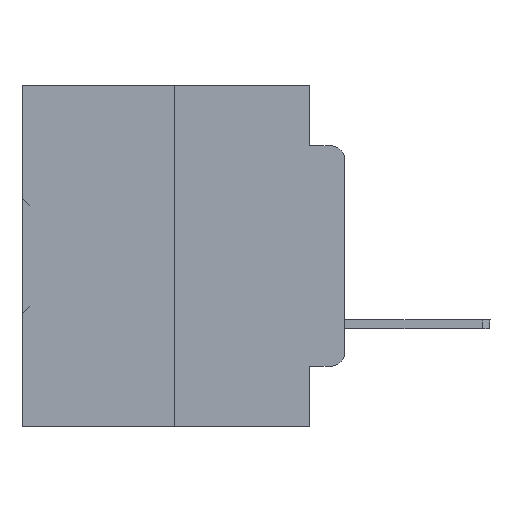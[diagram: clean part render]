
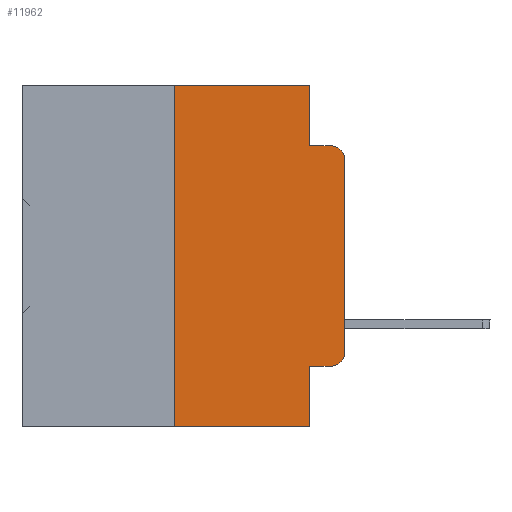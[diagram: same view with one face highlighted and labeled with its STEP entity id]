
A CAD part, left-side view. The second image highlights one B-rep face of the part: STEP entity #11962.
In plain terms, the highlighted planar face has unit normal (-1, 0, 0).
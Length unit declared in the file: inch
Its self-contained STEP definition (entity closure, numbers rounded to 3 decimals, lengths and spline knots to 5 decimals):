
#7 = PLANE ( 'NONE',  #31530 ) ;
#831 = VERTEX_POINT ( 'NONE', #22939 ) ;
#1155 = CARTESIAN_POINT ( 'NONE',  ( 0., 0.051, 0. ) ) ;
#1368 = EDGE_CURVE ( 'NONE', #8319, #36062, #19112, .T. ) ;
#2405 = DIRECTION ( 'NONE',  ( 0., 0., 1. ) ) ;
#2536 = DIRECTION ( 'NONE',  ( -1., 0., 0. ) ) ;
#2667 = CARTESIAN_POINT ( 'NONE',  ( 0., 0.051, -0.4115 ) ) ;
#2795 = LINE ( 'NONE', #1155, #24712 ) ;
#2955 = LINE ( 'NONE', #13779, #24870 ) ;
#3043 = ORIENTED_EDGE ( 'NONE', *, *, #25384, .F. ) ;
#3349 = VECTOR ( 'NONE', #2405, 39.37008 ) ;
#3354 = CARTESIAN_POINT ( 'NONE',  ( 0., 0.02, -0.0885 ) ) ;
#3370 = VERTEX_POINT ( 'NONE', #7289 ) ;
#4049 = VECTOR ( 'NONE', #7865, 39.37008 ) ;
#5136 = CARTESIAN_POINT ( 'NONE',  ( 0., 0.25, 0. ) ) ;
#6050 = LINE ( 'NONE', #37709, #29415 ) ;
#6312 = DIRECTION ( 'NONE',  ( -1., 0., 0. ) ) ;
#6445 = ORIENTED_EDGE ( 'NONE', *, *, #1368, .T. ) ;
#6804 = ORIENTED_EDGE ( 'NONE', *, *, #32723, .T. ) ;
#7289 = CARTESIAN_POINT ( 'NONE',  ( 0., 0., -0.1085 ) ) ;
#7563 = CIRCLE ( 'NONE', #25443, 0.02 ) ;
#7865 = DIRECTION ( 'NONE',  ( 0., -1., 0. ) ) ;
#8319 = VERTEX_POINT ( 'NONE', #31901 ) ;
#8374 = CARTESIAN_POINT ( 'NONE',  ( 0., 0.473, -0.5 ) ) ;
#9522 = CARTESIAN_POINT ( 'NONE',  ( 0., 0.02, -0.4115 ) ) ;
#9855 = VECTOR ( 'NONE', #17397, 39.37008 ) ;
#10699 = EDGE_CURVE ( 'NONE', #3370, #14332, #23942, .T. ) ;
#10856 = DIRECTION ( 'NONE',  ( 0., 0., 1. ) ) ;
#11103 = EDGE_CURVE ( 'NONE', #8319, #831, #38317, .T. ) ;
#11140 = VECTOR ( 'NONE', #23783, 39.37008 ) ;
#11633 = CARTESIAN_POINT ( 'NONE',  ( 0., 0.051, 0. ) ) ;
#11962 = ADVANCED_FACE ( 'NONE', ( #21568 ), #7, .F. ) ;
#12186 = AXIS2_PLACEMENT_3D ( 'NONE', #21081, #6312, #12460 ) ;
#12460 = DIRECTION ( 'NONE',  ( 0., 0., -1. ) ) ;
#12976 = EDGE_CURVE ( 'NONE', #22622, #14332, #6050, .T. ) ;
#13779 = CARTESIAN_POINT ( 'NONE',  ( 0., 0.25, 0. ) ) ;
#13898 = DIRECTION ( 'NONE',  ( 0., -1., 0. ) ) ;
#14332 = VERTEX_POINT ( 'NONE', #3354 ) ;
#14546 = CARTESIAN_POINT ( 'NONE',  ( 0., 0.02, -0.3915 ) ) ;
#15393 = DIRECTION ( 'NONE',  ( 0., 0., -1. ) ) ;
#15968 = CARTESIAN_POINT ( 'NONE',  ( 0., 0.473, 0. ) ) ;
#16521 = ORIENTED_EDGE ( 'NONE', *, *, #22679, .T. ) ;
#16950 = ORIENTED_EDGE ( 'NONE', *, *, #12976, .F. ) ;
#17397 = DIRECTION ( 'NONE',  ( 0., 0., -1. ) ) ;
#17766 = VERTEX_POINT ( 'NONE', #5136 ) ;
#18700 = DIRECTION ( 'NONE',  ( 0., -1., 0. ) ) ;
#18916 = ORIENTED_EDGE ( 'NONE', *, *, #32662, .T. ) ;
#19112 = LINE ( 'NONE', #2667, #11140 ) ;
#19905 = ORIENTED_EDGE ( 'NONE', *, *, #11103, .F. ) ;
#20248 = VERTEX_POINT ( 'NONE', #29637 ) ;
#20626 = ORIENTED_EDGE ( 'NONE', *, *, #10699, .T. ) ;
#21081 = CARTESIAN_POINT ( 'NONE',  ( 0., 0.02, -0.1085 ) ) ;
#21568 = FACE_OUTER_BOUND ( 'NONE', #21968, .T. ) ;
#21968 = EDGE_LOOP ( 'NONE', ( #6804, #20626, #16950, #22173, #34518, #3043, #16521, #19905, #6445, #18916 ) ) ;
#22173 = ORIENTED_EDGE ( 'NONE', *, *, #34942, .F. ) ;
#22622 = VERTEX_POINT ( 'NONE', #29134 ) ;
#22679 = EDGE_CURVE ( 'NONE', #27258, #831, #27880, .T. ) ;
#22939 = CARTESIAN_POINT ( 'NONE',  ( 0., 0.051, -0.5 ) ) ;
#22957 = LINE ( 'NONE', #38100, #3349 ) ;
#23378 = DIRECTION ( 'NONE',  ( 0., 0., -1. ) ) ;
#23734 = LINE ( 'NONE', #15968, #32088 ) ;
#23783 = DIRECTION ( 'NONE',  ( 0., -1., 0. ) ) ;
#23942 = CIRCLE ( 'NONE', #12186, 0.02 ) ;
#24497 = CARTESIAN_POINT ( 'NONE',  ( 0., 0.473, 0. ) ) ;
#24712 = VECTOR ( 'NONE', #28149, 39.37008 ) ;
#24870 = VECTOR ( 'NONE', #10856, 39.37008 ) ;
#25367 = CARTESIAN_POINT ( 'NONE',  ( 0., 0.25, -0.5 ) ) ;
#25384 = EDGE_CURVE ( 'NONE', #27258, #17766, #2955, .T. ) ;
#25443 = AXIS2_PLACEMENT_3D ( 'NONE', #14546, #2536, #23378 ) ;
#27258 = VERTEX_POINT ( 'NONE', #25367 ) ;
#27880 = LINE ( 'NONE', #8374, #4049 ) ;
#28149 = DIRECTION ( 'NONE',  ( 0., 0., -1. ) ) ;
#29134 = CARTESIAN_POINT ( 'NONE',  ( 0., 0.051, -0.0885 ) ) ;
#29228 = EDGE_CURVE ( 'NONE', #17766, #20248, #23734, .T. ) ;
#29415 = VECTOR ( 'NONE', #13898, 39.37008 ) ;
#29637 = CARTESIAN_POINT ( 'NONE',  ( 0., 0.051, 0. ) ) ;
#31530 = AXIS2_PLACEMENT_3D ( 'NONE', #24497, #33187, #15393 ) ;
#31901 = CARTESIAN_POINT ( 'NONE',  ( 0., 0.051, -0.4115 ) ) ;
#32088 = VECTOR ( 'NONE', #18700, 39.37008 ) ;
#32662 = EDGE_CURVE ( 'NONE', #36062, #32711, #7563, .T. ) ;
#32711 = VERTEX_POINT ( 'NONE', #38353 ) ;
#32723 = EDGE_CURVE ( 'NONE', #32711, #3370, #22957, .T. ) ;
#33187 = DIRECTION ( 'NONE',  ( 1., 0., 0. ) ) ;
#34518 = ORIENTED_EDGE ( 'NONE', *, *, #29228, .F. ) ;
#34942 = EDGE_CURVE ( 'NONE', #20248, #22622, #2795, .T. ) ;
#36062 = VERTEX_POINT ( 'NONE', #9522 ) ;
#37709 = CARTESIAN_POINT ( 'NONE',  ( 0., 0.051, -0.0885 ) ) ;
#38100 = CARTESIAN_POINT ( 'NONE',  ( 0., 0., 0. ) ) ;
#38317 = LINE ( 'NONE', #11633, #9855 ) ;
#38353 = CARTESIAN_POINT ( 'NONE',  ( 0., 0., -0.3915 ) ) ;
